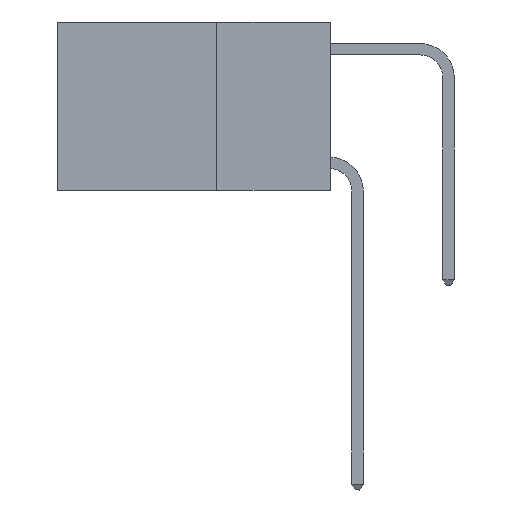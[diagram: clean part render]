
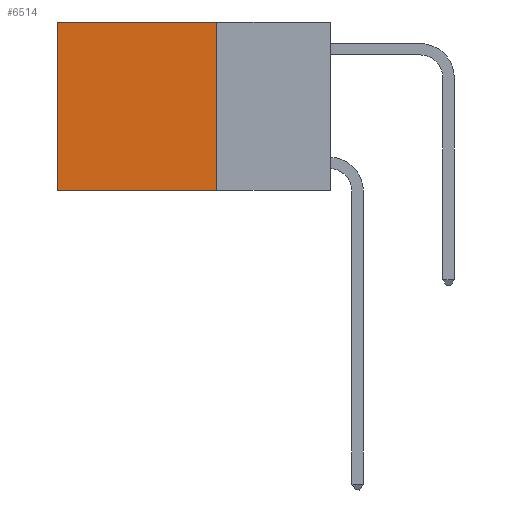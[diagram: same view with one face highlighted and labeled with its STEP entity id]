
A CAD part, left-side view. The second image highlights one B-rep face of the part: STEP entity #6514.
In plain terms, the highlighted planar face has unit normal (-1, 0, 0).
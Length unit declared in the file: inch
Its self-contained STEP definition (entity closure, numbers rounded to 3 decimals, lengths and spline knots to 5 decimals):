
#34 = VERTEX_POINT ( 'NONE', #3734 ) ;
#559 = VECTOR ( 'NONE', #17093, 39.37008 ) ;
#929 = VECTOR ( 'NONE', #7557, 39.37008 ) ;
#2384 = DIRECTION ( 'NONE',  ( 0., 0., -1. ) ) ;
#3734 = CARTESIAN_POINT ( 'NONE',  ( 0.2625, 0.6, 0. ) ) ;
#4442 = ORIENTED_EDGE ( 'NONE', *, *, #14576, .T. ) ;
#5417 = VERTEX_POINT ( 'NONE', #5921 ) ;
#5921 = CARTESIAN_POINT ( 'NONE',  ( 0.2625, 0.25, -0.37 ) ) ;
#6514 = ADVANCED_FACE ( 'NONE', ( #14219 ), #13014, .F. ) ;
#6673 = CARTESIAN_POINT ( 'NONE',  ( 0.2625, 0.6, 0. ) ) ;
#7557 = DIRECTION ( 'NONE',  ( 0., 1., 0. ) ) ;
#7645 = ORIENTED_EDGE ( 'NONE', *, *, #10594, .F. ) ;
#8222 = CARTESIAN_POINT ( 'NONE',  ( 0.2625, 0.25, 0. ) ) ;
#8353 = LINE ( 'NONE', #9839, #559 ) ;
#8652 = DIRECTION ( 'NONE',  ( 1., 0., 0. ) ) ;
#8928 = AXIS2_PLACEMENT_3D ( 'NONE', #17363, #8652, #18793 ) ;
#9132 = VECTOR ( 'NONE', #2384, 39.37008 ) ;
#9839 = CARTESIAN_POINT ( 'NONE',  ( 0.2625, 0.25, -0.37 ) ) ;
#10594 = EDGE_CURVE ( 'NONE', #5417, #15212, #8353, .T. ) ;
#11066 = DIRECTION ( 'NONE',  ( 0., 0., -1. ) ) ;
#11223 = LINE ( 'NONE', #6673, #15119 ) ;
#11288 = ORIENTED_EDGE ( 'NONE', *, *, #16158, .F. ) ;
#11726 = CARTESIAN_POINT ( 'NONE',  ( 0.2625, 0.25, 0. ) ) ;
#12128 = LINE ( 'NONE', #16312, #929 ) ;
#13014 = PLANE ( 'NONE',  #8928 ) ;
#13045 = LINE ( 'NONE', #8222, #9132 ) ;
#14176 = EDGE_CURVE ( 'NONE', #34, #15212, #11223, .T. ) ;
#14219 = FACE_OUTER_BOUND ( 'NONE', #18383, .T. ) ;
#14576 = EDGE_CURVE ( 'NONE', #17055, #34, #12128, .T. ) ;
#14955 = CARTESIAN_POINT ( 'NONE',  ( 0.2625, 0.6, -0.37 ) ) ;
#15119 = VECTOR ( 'NONE', #11066, 39.37008 ) ;
#15212 = VERTEX_POINT ( 'NONE', #14955 ) ;
#16158 = EDGE_CURVE ( 'NONE', #17055, #5417, #13045, .T. ) ;
#16312 = CARTESIAN_POINT ( 'NONE',  ( 0.2625, 0.25, 0. ) ) ;
#17055 = VERTEX_POINT ( 'NONE', #11726 ) ;
#17093 = DIRECTION ( 'NONE',  ( 0., 1., 0. ) ) ;
#17363 = CARTESIAN_POINT ( 'NONE',  ( 0.2625, 0.25, 0. ) ) ;
#18383 = EDGE_LOOP ( 'NONE', ( #18787, #7645, #11288, #4442 ) ) ;
#18787 = ORIENTED_EDGE ( 'NONE', *, *, #14176, .T. ) ;
#18793 = DIRECTION ( 'NONE',  ( 0., 0., -1. ) ) ;
